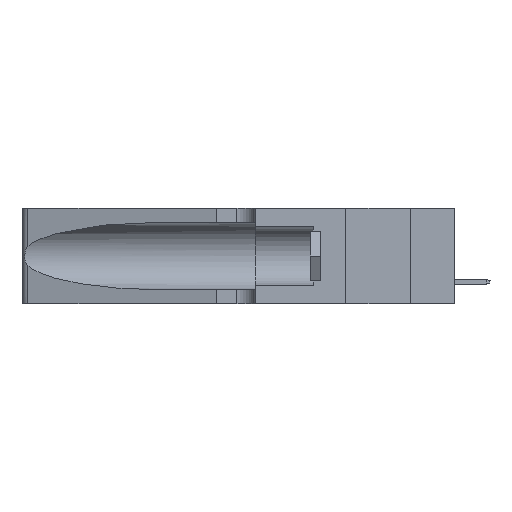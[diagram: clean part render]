
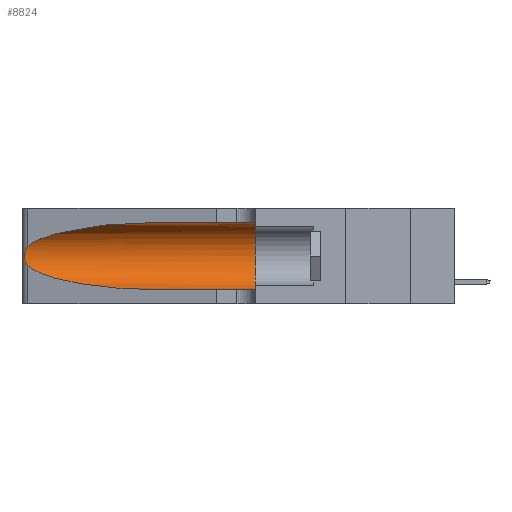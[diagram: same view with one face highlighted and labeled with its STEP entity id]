
A CAD part, left-side view. The second image highlights one B-rep face of the part: STEP entity #8824.
In plain terms, the highlighted cylindrical face has radius 3.308 mm (diameter 6.617 mm), a partial arc.
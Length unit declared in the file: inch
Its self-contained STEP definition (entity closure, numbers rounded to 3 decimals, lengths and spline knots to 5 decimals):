
#1173 = FACE_OUTER_BOUND ( 'NONE', #5707, .T. ) ;
#1542 = EDGE_CURVE ( 'NONE', #28763, #18703, #27982, .T. ) ;
#1635 = CARTESIAN_POINT ( 'NONE',  ( 0.1305, 0.72297, 0.31525 ) ) ;
#1703 = CARTESIAN_POINT ( 'NONE',  ( 0.25787, 1.23484, 0.2124 ) ) ;
#1711 = CARTESIAN_POINT ( 'NONE',  ( 0.1305, 0.35, 0.05475 ) ) ;
#1836 = CARTESIAN_POINT ( 'NONE',  ( 0.26075, 1.23896, 0.178 ) ) ;
#3404 = CARTESIAN_POINT ( 'NONE',  ( 0.25487, 1.22718, 0.14631 ) ) ;
#4349 = VECTOR ( 'NONE', #23054, 39.37008 ) ;
#5081 = CARTESIAN_POINT ( 'NONE',  ( 0.25487, 1.22718, 0.22369 ) ) ;
#5327 = CARTESIAN_POINT ( 'NONE',  ( 0.2373, 1.15595, 0.08982 ) ) ;
#5707 = EDGE_LOOP ( 'NONE', ( #21056, #7061, #7794, #16475, #13232, #10208 ) ) ;
#5881 = CARTESIAN_POINT ( 'NONE',  ( 0.1305, 1.61858, 0.185 ) ) ;
#6163 = CYLINDRICAL_SURFACE ( 'NONE', #15128, 0.13025 ) ;
#6179 = LINE ( 'NONE', #12968, #22070 ) ;
#6319 = CARTESIAN_POINT ( 'NONE',  ( 0.25487, 1.22718, 0.22369 ) ) ;
#6663 = CARTESIAN_POINT ( 'NONE',  ( 0.26075, 1.23896, 0.19203 ) ) ;
#6822 = CARTESIAN_POINT ( 'NONE',  ( 0.1305, 0.35, 0.31525 ) ) ;
#6877 = CARTESIAN_POINT ( 'NONE',  ( 0.1305, 1.61858, 0.05475 ) ) ;
#6905 = EDGE_CURVE ( 'NONE', #13647, #23619, #9985, .T. ) ;
#7061 = ORIENTED_EDGE ( 'NONE', *, *, #13074, .T. ) ;
#7794 = ORIENTED_EDGE ( 'NONE', *, *, #6905, .T. ) ;
#7803 = AXIS2_PLACEMENT_3D ( 'NONE', #23301, #27841, #25670 ) ;
#8248 = CARTESIAN_POINT ( 'NONE',  ( 0.2373, 1.15595, 0.28018 ) ) ;
#8824 = ADVANCED_FACE ( 'NONE', ( #1173 ), #6163, .F. ) ;
#9985 =( BOUNDED_CURVE ( )  B_SPLINE_CURVE ( 3, ( #23266, #5327, #22820, #20619 ),
 .UNSPECIFIED., .F., .F. ) 
 B_SPLINE_CURVE_WITH_KNOTS ( ( 4, 4 ),
 ( 3.44316, 4.71239 ),
 .UNSPECIFIED. ) 
 CURVE ( )  GEOMETRIC_REPRESENTATION_ITEM ( )  RATIONAL_B_SPLINE_CURVE ( ( 1., 0.87, 0.87, 1. ) ) 
 REPRESENTATION_ITEM ( '' )  );
#10208 = ORIENTED_EDGE ( 'NONE', *, *, #25056, .F. ) ;
#10591 = DIRECTION ( 'NONE',  ( 0., -1., 0. ) ) ;
#10813 = CARTESIAN_POINT ( 'NONE',  ( 0.26017, 1.23833, 0.17102 ) ) ;
#10957 = CARTESIAN_POINT ( 'NONE',  ( 0.25789, 1.23486, 0.15765 ) ) ;
#11043 = EDGE_CURVE ( 'NONE', #23619, #18703, #12050, .T. ) ;
#11109 = CARTESIAN_POINT ( 'NONE',  ( 0.25555, 1.22994, 0.2215 ) ) ;
#12050 = LINE ( 'NONE', #6877, #4349 ) ;
#12373 = DIRECTION ( 'NONE',  ( 0., 0., -1. ) ) ;
#12968 = CARTESIAN_POINT ( 'NONE',  ( 0.1305, 1.61858, 0.31525 ) ) ;
#13028 = CARTESIAN_POINT ( 'NONE',  ( 0.25487, 1.22718, 0.22369 ) ) ;
#13074 = EDGE_CURVE ( 'NONE', #21317, #13647, #15873, .T. ) ;
#13232 = ORIENTED_EDGE ( 'NONE', *, *, #1542, .F. ) ;
#13461 = CARTESIAN_POINT ( 'NONE',  ( 0.25487, 1.22718, 0.14631 ) ) ;
#13647 = VERTEX_POINT ( 'NONE', #3404 ) ;
#13874 = EDGE_CURVE ( 'NONE', #14420, #21317, #15230, .T. ) ;
#14420 = VERTEX_POINT ( 'NONE', #27943 ) ;
#15128 = AXIS2_PLACEMENT_3D ( 'NONE', #5881, #10591, #12373 ) ;
#15230 =( BOUNDED_CURVE ( )  B_SPLINE_CURVE ( 3, ( #1635, #28947, #8248, #6319 ),
 .UNSPECIFIED., .F., .F. ) 
 B_SPLINE_CURVE_WITH_KNOTS ( ( 4, 4 ),
 ( 1.5708, 2.84003 ),
 .UNSPECIFIED. ) 
 CURVE ( )  GEOMETRIC_REPRESENTATION_ITEM ( )  RATIONAL_B_SPLINE_CURVE ( ( 1., 0.87, 0.87, 1. ) ) 
 REPRESENTATION_ITEM ( '' )  );
#15663 = CARTESIAN_POINT ( 'NONE',  ( 0.25555, 1.22993, 0.14849 ) ) ;
#15873 = B_SPLINE_CURVE_WITH_KNOTS ( 'NONE', 3,
 ( #13028, #11109, #20056, #1703, #19633, #26808, #6663, #1836, #10813, #24628, #10957, #28732, #15663, #13461 ),
 .UNSPECIFIED., .F., .F.,
 ( 4, 2, 2, 2, 2, 2, 4 ),
 ( 0., 0.00027, 0.00053, 0.00107, 0.0016, 0.00187, 0.00214 ),
 .UNSPECIFIED. ) ;
#16475 = ORIENTED_EDGE ( 'NONE', *, *, #11043, .T. ) ;
#18703 = VERTEX_POINT ( 'NONE', #1711 ) ;
#19633 = CARTESIAN_POINT ( 'NONE',  ( 0.25854, 1.2359, 0.20912 ) ) ;
#20056 = CARTESIAN_POINT ( 'NONE',  ( 0.25639, 1.23184, 0.21858 ) ) ;
#20619 = CARTESIAN_POINT ( 'NONE',  ( 0.1305, 0.72297, 0.05475 ) ) ;
#21056 = ORIENTED_EDGE ( 'NONE', *, *, #13874, .T. ) ;
#21317 = VERTEX_POINT ( 'NONE', #5081 ) ;
#21904 = DIRECTION ( 'NONE',  ( 0., -1., 0. ) ) ;
#22070 = VECTOR ( 'NONE', #21904, 39.37008 ) ;
#22820 = CARTESIAN_POINT ( 'NONE',  ( 0.18966, 0.96281, 0.05475 ) ) ;
#23054 = DIRECTION ( 'NONE',  ( 0., -1., 0. ) ) ;
#23266 = CARTESIAN_POINT ( 'NONE',  ( 0.25487, 1.22718, 0.14631 ) ) ;
#23301 = CARTESIAN_POINT ( 'NONE',  ( 0.1305, 0.35, 0.185 ) ) ;
#23543 = CARTESIAN_POINT ( 'NONE',  ( 0.1305, 0.72297, 0.05475 ) ) ;
#23619 = VERTEX_POINT ( 'NONE', #23543 ) ;
#24628 = CARTESIAN_POINT ( 'NONE',  ( 0.25856, 1.23593, 0.16098 ) ) ;
#25056 = EDGE_CURVE ( 'NONE', #14420, #28763, #6179, .T. ) ;
#25670 = DIRECTION ( 'NONE',  ( 0., 0., 1. ) ) ;
#26808 = CARTESIAN_POINT ( 'NONE',  ( 0.26018, 1.23835, 0.19895 ) ) ;
#27841 = DIRECTION ( 'NONE',  ( 0., 1., 0. ) ) ;
#27943 = CARTESIAN_POINT ( 'NONE',  ( 0.1305, 0.72297, 0.31525 ) ) ;
#27982 = CIRCLE ( 'NONE', #7803, 0.13025 ) ;
#28732 = CARTESIAN_POINT ( 'NONE',  ( 0.25639, 1.23186, 0.15144 ) ) ;
#28763 = VERTEX_POINT ( 'NONE', #6822 ) ;
#28947 = CARTESIAN_POINT ( 'NONE',  ( 0.18966, 0.96281, 0.31525 ) ) ;
